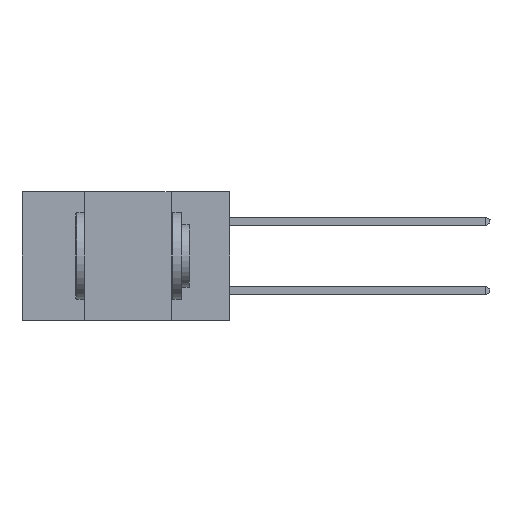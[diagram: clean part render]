
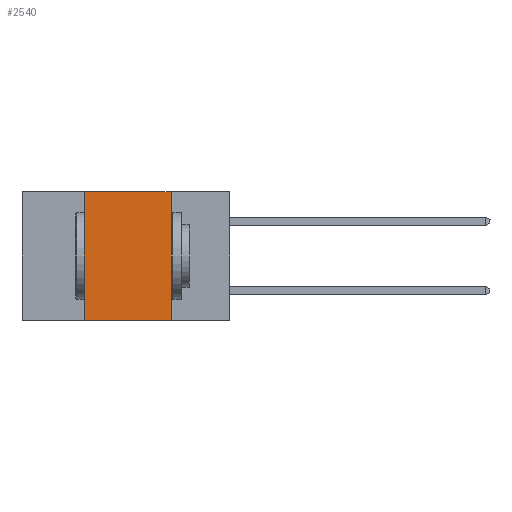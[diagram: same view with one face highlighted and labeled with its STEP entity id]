
A CAD part, left-side view. The second image highlights one B-rep face of the part: STEP entity #2540.
In plain terms, the highlighted planar face has unit normal (-1, 0, 0).
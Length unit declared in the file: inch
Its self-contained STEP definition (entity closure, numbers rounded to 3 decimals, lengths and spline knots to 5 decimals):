
#332 = EDGE_CURVE ( 'NONE', #7203, #9637, #9595, .T. ) ;
#817 = DIRECTION ( 'NONE',  ( 0., 0., -1. ) ) ;
#939 = LINE ( 'NONE', #12379, #8095 ) ;
#1331 = VECTOR ( 'NONE', #3123, 39.37008 ) ;
#1714 = EDGE_CURVE ( 'NONE', #7074, #10522, #3363, .T. ) ;
#2250 = CARTESIAN_POINT ( 'NONE',  ( 0., 0.42, -0.37 ) ) ;
#2526 = FACE_OUTER_BOUND ( 'NONE', #6989, .T. ) ;
#2540 = ADVANCED_FACE ( 'NONE', ( #2526 ), #11095, .F. ) ;
#2803 = DIRECTION ( 'NONE',  ( 1., 0., 0. ) ) ;
#3123 = DIRECTION ( 'NONE',  ( 0., -1., 0. ) ) ;
#3317 = DIRECTION ( 'NONE',  ( 0., 0., 1. ) ) ;
#3341 = EDGE_CURVE ( 'NONE', #9637, #7074, #939, .T. ) ;
#3363 = LINE ( 'NONE', #5792, #13468 ) ;
#4846 = DIRECTION ( 'NONE',  ( 0., 0., -1. ) ) ;
#5254 = CARTESIAN_POINT ( 'NONE',  ( 0., 0.42, 0. ) ) ;
#5712 = CARTESIAN_POINT ( 'NONE',  ( 0., 0.17, -0.37 ) ) ;
#5792 = CARTESIAN_POINT ( 'NONE',  ( 0., 0.17, 0. ) ) ;
#5796 = LINE ( 'NONE', #8596, #1331 ) ;
#6308 = CARTESIAN_POINT ( 'NONE',  ( 0., 0.17, 0. ) ) ;
#6644 = EDGE_CURVE ( 'NONE', #7203, #10522, #5796, .T. ) ;
#6750 = VECTOR ( 'NONE', #3317, 39.37008 ) ;
#6989 = EDGE_LOOP ( 'NONE', ( #10725, #11540, #8222, #9491 ) ) ;
#7074 = VERTEX_POINT ( 'NONE', #6308 ) ;
#7203 = VERTEX_POINT ( 'NONE', #2250 ) ;
#7927 = CARTESIAN_POINT ( 'NONE',  ( 0., 0.42, 0. ) ) ;
#8095 = VECTOR ( 'NONE', #9204, 39.37008 ) ;
#8222 = ORIENTED_EDGE ( 'NONE', *, *, #332, .F. ) ;
#8596 = CARTESIAN_POINT ( 'NONE',  ( 0., 0.6, -0.37 ) ) ;
#8981 = CARTESIAN_POINT ( 'NONE',  ( 0., 0.6, 0. ) ) ;
#9204 = DIRECTION ( 'NONE',  ( 0., -1., 0. ) ) ;
#9491 = ORIENTED_EDGE ( 'NONE', *, *, #6644, .T. ) ;
#9595 = LINE ( 'NONE', #5254, #6750 ) ;
#9637 = VERTEX_POINT ( 'NONE', #7927 ) ;
#10522 = VERTEX_POINT ( 'NONE', #5712 ) ;
#10725 = ORIENTED_EDGE ( 'NONE', *, *, #1714, .F. ) ;
#11095 = PLANE ( 'NONE',  #12059 ) ;
#11540 = ORIENTED_EDGE ( 'NONE', *, *, #3341, .F. ) ;
#12059 = AXIS2_PLACEMENT_3D ( 'NONE', #8981, #2803, #817 ) ;
#12379 = CARTESIAN_POINT ( 'NONE',  ( 0., 0.6, 0. ) ) ;
#13468 = VECTOR ( 'NONE', #4846, 39.37008 ) ;
